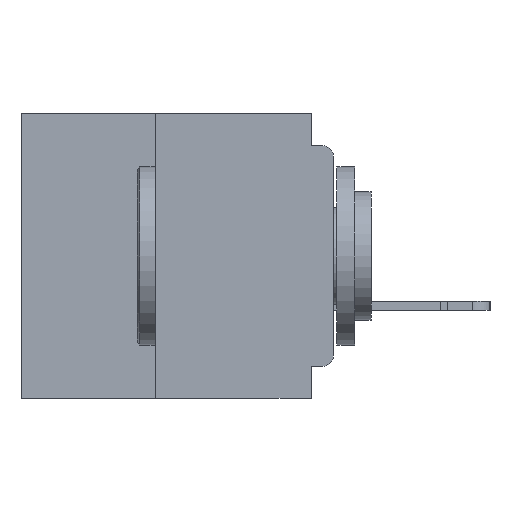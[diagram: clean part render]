
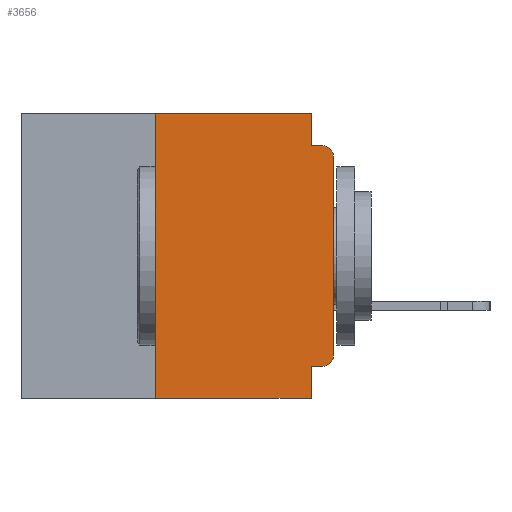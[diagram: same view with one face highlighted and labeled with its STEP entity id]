
A CAD part, left-side view. The second image highlights one B-rep face of the part: STEP entity #3656.
In plain terms, the highlighted planar face has unit normal (-1, 0, 0).
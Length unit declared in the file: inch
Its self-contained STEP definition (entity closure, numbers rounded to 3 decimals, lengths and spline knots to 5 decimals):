
#2222 = VECTOR ( 'NONE', #19861, 39.37008 ) ;
#2865 = EDGE_CURVE ( 'NONE', #22255, #9641, #55799, .T. ) ;
#3656 = ADVANCED_FACE ( 'NONE', ( #45143 ), #26544, .F. ) ;
#5849 = DIRECTION ( 'NONE',  ( 0., 0., -1. ) ) ;
#8369 = EDGE_CURVE ( 'NONE', #36073, #45331, #42162, .T. ) ;
#8381 = LINE ( 'NONE', #42589, #32718 ) ;
#8435 = LINE ( 'NONE', #33504, #34412 ) ;
#9641 = VERTEX_POINT ( 'NONE', #36816 ) ;
#10774 = DIRECTION ( 'NONE',  ( 0., 0., 1. ) ) ;
#10916 = DIRECTION ( 'NONE',  ( 0., 0., 1. ) ) ;
#11253 = VECTOR ( 'NONE', #10916, 39.37008 ) ;
#11599 = EDGE_CURVE ( 'NONE', #45331, #33415, #8435, .T. ) ;
#12059 = EDGE_CURVE ( 'NONE', #36073, #9641, #8381, .T. ) ;
#13257 = CARTESIAN_POINT ( 'NONE',  ( 0., 0., -0.34 ) ) ;
#13498 = LINE ( 'NONE', #62471, #39460 ) ;
#15047 = VERTEX_POINT ( 'NONE', #33234 ) ;
#16206 = VERTEX_POINT ( 'NONE', #31985 ) ;
#17062 = EDGE_CURVE ( 'NONE', #40875, #61032, #58025, .T. ) ;
#17603 = AXIS2_PLACEMENT_3D ( 'NONE', #29927, #66197, #35122 ) ;
#18391 = LINE ( 'NONE', #24009, #20027 ) ;
#19100 = ORIENTED_EDGE ( 'NONE', *, *, #32008, .F. ) ;
#19861 = DIRECTION ( 'NONE',  ( 0., 0., -1. ) ) ;
#20027 = VECTOR ( 'NONE', #39376, 39.37008 ) ;
#21642 = ORIENTED_EDGE ( 'NONE', *, *, #66391, .F. ) ;
#22255 = VERTEX_POINT ( 'NONE', #38669 ) ;
#23686 = VECTOR ( 'NONE', #42889, 39.37008 ) ;
#24009 = CARTESIAN_POINT ( 'NONE',  ( 0., 0., -0.355 ) ) ;
#24341 = VECTOR ( 'NONE', #10774, 39.37008 ) ;
#25089 = ORIENTED_EDGE ( 'NONE', *, *, #11599, .F. ) ;
#25659 = DIRECTION ( 'NONE',  ( -1., 0., 0. ) ) ;
#26544 = PLANE ( 'NONE',  #56565 ) ;
#27890 = CARTESIAN_POINT ( 'NONE',  ( 0., 0.031, 0. ) ) ;
#28163 = AXIS2_PLACEMENT_3D ( 'NONE', #56715, #25659, #61879 ) ;
#28350 = DIRECTION ( 'NONE',  ( 0., -1., 0. ) ) ;
#29927 = CARTESIAN_POINT ( 'NONE',  ( 0., 0.015, -0.06 ) ) ;
#30714 = CARTESIAN_POINT ( 'NONE',  ( 0., 0.015, -0.355 ) ) ;
#30725 = ORIENTED_EDGE ( 'NONE', *, *, #17062, .T. ) ;
#31413 = DIRECTION ( 'NONE',  ( 0., -1., 0. ) ) ;
#31985 = CARTESIAN_POINT ( 'NONE',  ( 0., 0.015, -0.045 ) ) ;
#32008 = EDGE_CURVE ( 'NONE', #50213, #16206, #13498, .T. ) ;
#32718 = VECTOR ( 'NONE', #47775, 39.37008 ) ;
#33234 = CARTESIAN_POINT ( 'NONE',  ( 0., 0., -0.06 ) ) ;
#33415 = VERTEX_POINT ( 'NONE', #27890 ) ;
#33504 = CARTESIAN_POINT ( 'NONE',  ( 0., 0.437, 0. ) ) ;
#33684 = CARTESIAN_POINT ( 'NONE',  ( 0., 0.031, -0.045 ) ) ;
#34412 = VECTOR ( 'NONE', #28350, 39.37008 ) ;
#35122 = DIRECTION ( 'NONE',  ( 0., 0., -1. ) ) ;
#35463 = CARTESIAN_POINT ( 'NONE',  ( 0., 0.031, -0.4 ) ) ;
#36073 = VERTEX_POINT ( 'NONE', #41389 ) ;
#36442 = LINE ( 'NONE', #41889, #24341 ) ;
#36816 = CARTESIAN_POINT ( 'NONE',  ( 0., 0.031, -0.4 ) ) ;
#36922 = DIRECTION ( 'NONE',  ( 1., 0., 0. ) ) ;
#38669 = CARTESIAN_POINT ( 'NONE',  ( 0., 0.031, -0.355 ) ) ;
#39376 = DIRECTION ( 'NONE',  ( 0., 1., 0. ) ) ;
#39460 = VECTOR ( 'NONE', #31413, 39.37008 ) ;
#40875 = VERTEX_POINT ( 'NONE', #30714 ) ;
#41389 = CARTESIAN_POINT ( 'NONE',  ( 0., 0.25, -0.4 ) ) ;
#41808 = EDGE_LOOP ( 'NONE', ( #64875, #52402, #19100, #21642, #25089, #63840, #62275, #52058, #64048, #30725 ) ) ;
#41889 = CARTESIAN_POINT ( 'NONE',  ( 0., 0., 0. ) ) ;
#42162 = LINE ( 'NONE', #52454, #11253 ) ;
#42589 = CARTESIAN_POINT ( 'NONE',  ( 0., 0.437, -0.4 ) ) ;
#42661 = CARTESIAN_POINT ( 'NONE',  ( 0., 0.031, 0. ) ) ;
#42889 = DIRECTION ( 'NONE',  ( 0., 0., -1. ) ) ;
#44592 = EDGE_CURVE ( 'NONE', #61032, #15047, #36442, .T. ) ;
#45143 = FACE_OUTER_BOUND ( 'NONE', #41808, .T. ) ;
#45331 = VERTEX_POINT ( 'NONE', #53623 ) ;
#47181 = CARTESIAN_POINT ( 'NONE',  ( 0., 0.437, 0. ) ) ;
#47775 = DIRECTION ( 'NONE',  ( 0., -1., 0. ) ) ;
#50213 = VERTEX_POINT ( 'NONE', #33684 ) ;
#51234 = LINE ( 'NONE', #42661, #23686 ) ;
#52058 = ORIENTED_EDGE ( 'NONE', *, *, #2865, .F. ) ;
#52402 = ORIENTED_EDGE ( 'NONE', *, *, #64409, .T. ) ;
#52454 = CARTESIAN_POINT ( 'NONE',  ( 0., 0.25, -0.4 ) ) ;
#53623 = CARTESIAN_POINT ( 'NONE',  ( 0., 0.25, 0. ) ) ;
#55799 = LINE ( 'NONE', #35463, #2222 ) ;
#56565 = AXIS2_PLACEMENT_3D ( 'NONE', #47181, #36922, #5849 ) ;
#56715 = CARTESIAN_POINT ( 'NONE',  ( 0., 0.015, -0.34 ) ) ;
#58025 = CIRCLE ( 'NONE', #28163, 0.015 ) ;
#58695 = EDGE_CURVE ( 'NONE', #40875, #22255, #18391, .T. ) ;
#60444 = CIRCLE ( 'NONE', #17603, 0.015 ) ;
#61032 = VERTEX_POINT ( 'NONE', #13257 ) ;
#61879 = DIRECTION ( 'NONE',  ( 0., 0., -1. ) ) ;
#62275 = ORIENTED_EDGE ( 'NONE', *, *, #12059, .T. ) ;
#62471 = CARTESIAN_POINT ( 'NONE',  ( 0., 0., -0.045 ) ) ;
#63840 = ORIENTED_EDGE ( 'NONE', *, *, #8369, .F. ) ;
#64048 = ORIENTED_EDGE ( 'NONE', *, *, #58695, .F. ) ;
#64409 = EDGE_CURVE ( 'NONE', #15047, #16206, #60444, .T. ) ;
#64875 = ORIENTED_EDGE ( 'NONE', *, *, #44592, .T. ) ;
#66197 = DIRECTION ( 'NONE',  ( -1., 0., 0. ) ) ;
#66391 = EDGE_CURVE ( 'NONE', #33415, #50213, #51234, .T. ) ;
